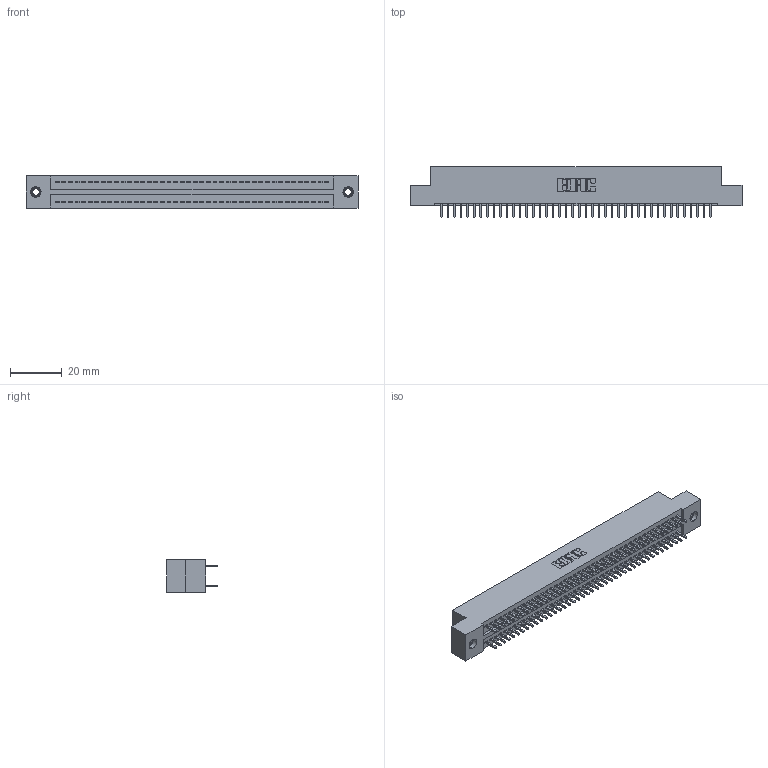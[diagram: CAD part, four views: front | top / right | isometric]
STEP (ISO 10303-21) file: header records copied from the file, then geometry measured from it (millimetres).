
FILE_DESCRIPTION (( 'STEP AP203' ), '1' );
FILE_NAME ('325-084-520-207.STEP', '2020-02-25T05:02:17', ( '' ), ( '' ), 'SwSTEP 2.0', 'SolidWorks 2016', '' );
FILE_SCHEMA (( 'CONFIG_CONTROL_DESIGN' ));
Length unit declared in the file: inch
Products named in the file (4): 325 Part_TI; 325-084-520-207; 345-250-001_345-250-005-103; 325-292-001_325-293-120
Assembly tree (87 placements, depth 2):
  325-084-520-207
    325 Part_TI
    325-292-001_325-293-120  x84
    345-250-001_345-250-005-103  x2
Bounding box: 128.4 x 19.68 x 12.45 mm (x, y, z)
Volume: 16549.4 mm3; surface area: 19887.3 mm2
Topology: 87 solids, 87 shells, 4542 faces, 13467 edges, 8858 vertices
Faces by surface type: plane 3126, cylinder 1400, cone 12, torus 4
Entity records: 28224 total; most frequent: CARTESIAN_POINT 4661, ORIENTED_EDGE 4590, DIRECTION 4013, EDGE_CURVE 2295, LINE 2147, VECTOR 2147, VERTEX_POINT 1524, AXIS2_PLACEMENT_3D 933
